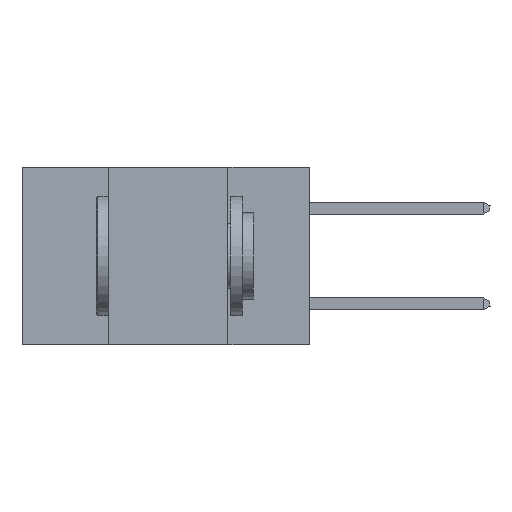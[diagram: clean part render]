
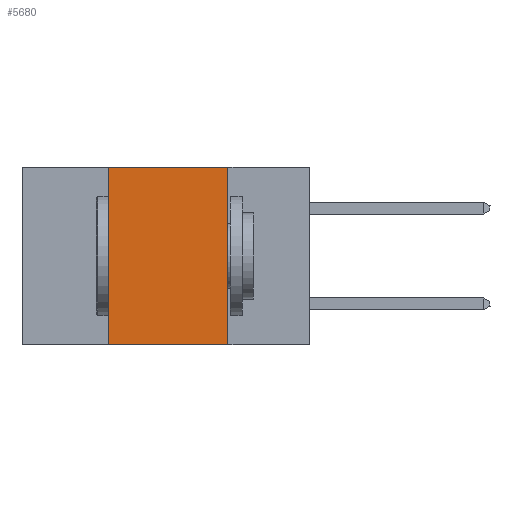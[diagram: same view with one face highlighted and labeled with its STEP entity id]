
A CAD part, left-side view. The second image highlights one B-rep face of the part: STEP entity #5680.
In plain terms, the highlighted planar face has unit normal (-1, 0, 0).
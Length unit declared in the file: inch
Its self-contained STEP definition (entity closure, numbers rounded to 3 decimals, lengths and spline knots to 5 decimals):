
#556 = CARTESIAN_POINT ( 'NONE',  ( 0., 0.42, 0. ) ) ;
#1153 = EDGE_LOOP ( 'NONE', ( #9872, #10544, #9684, #14755 ) ) ;
#1320 = EDGE_CURVE ( 'NONE', #4143, #14437, #16593, .T. ) ;
#2936 = DIRECTION ( 'NONE',  ( 0., 0., -1. ) ) ;
#3032 = CARTESIAN_POINT ( 'NONE',  ( 0., 0.17, 0. ) ) ;
#3046 = LINE ( 'NONE', #11897, #5855 ) ;
#3919 = VECTOR ( 'NONE', #5802, 39.37008 ) ;
#4143 = VERTEX_POINT ( 'NONE', #12196 ) ;
#4237 = VERTEX_POINT ( 'NONE', #11163 ) ;
#4244 = CARTESIAN_POINT ( 'NONE',  ( 0., 0.6, 0. ) ) ;
#5302 = DIRECTION ( 'NONE',  ( 0., 0., -1. ) ) ;
#5403 = LINE ( 'NONE', #10291, #15171 ) ;
#5680 = ADVANCED_FACE ( 'NONE', ( #11589 ), #9592, .F. ) ;
#5802 = DIRECTION ( 'NONE',  ( 0., 0., 1. ) ) ;
#5855 = VECTOR ( 'NONE', #13156, 39.37008 ) ;
#6600 = VERTEX_POINT ( 'NONE', #556 ) ;
#7558 = LINE ( 'NONE', #15959, #3919 ) ;
#8430 = CARTESIAN_POINT ( 'NONE',  ( 0., 0.17, -0.37 ) ) ;
#9592 = PLANE ( 'NONE',  #15035 ) ;
#9684 = ORIENTED_EDGE ( 'NONE', *, *, #15082, .F. ) ;
#9872 = ORIENTED_EDGE ( 'NONE', *, *, #1320, .F. ) ;
#10291 = CARTESIAN_POINT ( 'NONE',  ( 0., 0.6, -0.37 ) ) ;
#10544 = ORIENTED_EDGE ( 'NONE', *, *, #15583, .F. ) ;
#10836 = DIRECTION ( 'NONE',  ( 1., 0., 0. ) ) ;
#11163 = CARTESIAN_POINT ( 'NONE',  ( 0., 0.42, -0.37 ) ) ;
#11540 = DIRECTION ( 'NONE',  ( 0., -1., 0. ) ) ;
#11589 = FACE_OUTER_BOUND ( 'NONE', #1153, .T. ) ;
#11897 = CARTESIAN_POINT ( 'NONE',  ( 0., 0.6, 0. ) ) ;
#12196 = CARTESIAN_POINT ( 'NONE',  ( 0., 0.17, 0. ) ) ;
#13156 = DIRECTION ( 'NONE',  ( 0., -1., 0. ) ) ;
#14437 = VERTEX_POINT ( 'NONE', #8430 ) ;
#14755 = ORIENTED_EDGE ( 'NONE', *, *, #16044, .T. ) ;
#15035 = AXIS2_PLACEMENT_3D ( 'NONE', #4244, #10836, #2936 ) ;
#15082 = EDGE_CURVE ( 'NONE', #4237, #6600, #7558, .T. ) ;
#15171 = VECTOR ( 'NONE', #11540, 39.37008 ) ;
#15583 = EDGE_CURVE ( 'NONE', #6600, #4143, #3046, .T. ) ;
#15959 = CARTESIAN_POINT ( 'NONE',  ( 0., 0.42, 0. ) ) ;
#16044 = EDGE_CURVE ( 'NONE', #4237, #14437, #5403, .T. ) ;
#16199 = VECTOR ( 'NONE', #5302, 39.37008 ) ;
#16593 = LINE ( 'NONE', #3032, #16199 ) ;
